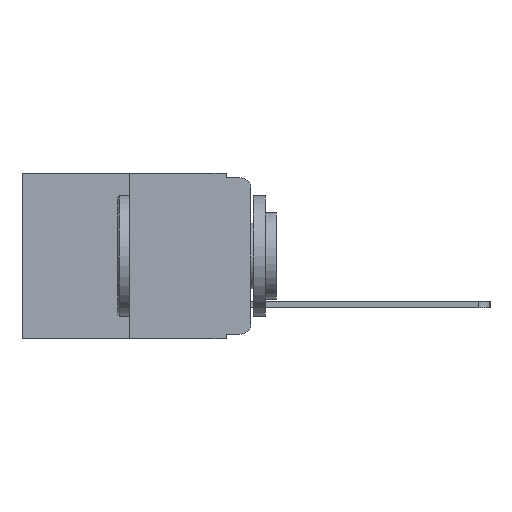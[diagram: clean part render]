
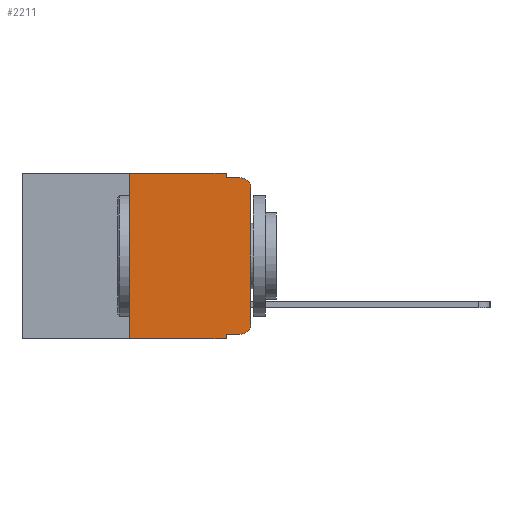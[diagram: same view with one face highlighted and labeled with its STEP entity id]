
A CAD part, left-side view. The second image highlights one B-rep face of the part: STEP entity #2211.
In plain terms, the highlighted planar face has unit normal (-1, 0, 0).
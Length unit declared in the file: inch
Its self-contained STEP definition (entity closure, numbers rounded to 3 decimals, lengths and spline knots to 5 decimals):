
#130 = CARTESIAN_POINT ( 'NONE',  ( 0., 0.473, 0. ) ) ;
#476 = DIRECTION ( 'NONE',  ( -1., 0., 0. ) ) ;
#540 = VECTOR ( 'NONE', #4897, 39.37008 ) ;
#891 = ORIENTED_EDGE ( 'NONE', *, *, #9728, .T. ) ;
#902 = LINE ( 'NONE', #9232, #6097 ) ;
#924 = VERTEX_POINT ( 'NONE', #2674 ) ;
#1056 = CIRCLE ( 'NONE', #1705, 0.02 ) ;
#1134 = VERTEX_POINT ( 'NONE', #9657 ) ;
#1220 = LINE ( 'NONE', #130, #8833 ) ;
#1580 = VECTOR ( 'NONE', #7499, 39.37008 ) ;
#1705 = AXIS2_PLACEMENT_3D ( 'NONE', #10366, #5227, #11197 ) ;
#1789 = DIRECTION ( 'NONE',  ( 0., 0., -1. ) ) ;
#2211 = ADVANCED_FACE ( 'NONE', ( #8863 ), #8914, .F. ) ;
#2260 = VECTOR ( 'NONE', #2673, 39.37008 ) ;
#2673 = DIRECTION ( 'NONE',  ( 0., 0., 1. ) ) ;
#2674 = CARTESIAN_POINT ( 'NONE',  ( 0., 0.051, -0.01 ) ) ;
#2981 = ORIENTED_EDGE ( 'NONE', *, *, #9771, .F. ) ;
#3163 = VECTOR ( 'NONE', #7651, 39.37008 ) ;
#3220 = VERTEX_POINT ( 'NONE', #5065 ) ;
#3433 = CARTESIAN_POINT ( 'NONE',  ( 0., 0.25, -0.343 ) ) ;
#3993 = CARTESIAN_POINT ( 'NONE',  ( 0., 0.051, 0. ) ) ;
#4006 = EDGE_LOOP ( 'NONE', ( #891, #9384, #2981, #10443, #7419, #5955, #8093, #11116, #12118, #6270 ) ) ;
#4471 = VERTEX_POINT ( 'NONE', #10386 ) ;
#4511 = DIRECTION ( 'NONE',  ( 0., -1., 0. ) ) ;
#4897 = DIRECTION ( 'NONE',  ( 0., 0., 1. ) ) ;
#4905 = AXIS2_PLACEMENT_3D ( 'NONE', #5896, #8942, #1789 ) ;
#5065 = CARTESIAN_POINT ( 'NONE',  ( 0., 0., -0.03 ) ) ;
#5227 = DIRECTION ( 'NONE',  ( -1., 0., 0. ) ) ;
#5720 = CARTESIAN_POINT ( 'NONE',  ( 0., 0., -0.313 ) ) ;
#5896 = CARTESIAN_POINT ( 'NONE',  ( 0., 0.473, 0. ) ) ;
#5947 = CARTESIAN_POINT ( 'NONE',  ( 0., 0.473, -0.343 ) ) ;
#5955 = ORIENTED_EDGE ( 'NONE', *, *, #9822, .F. ) ;
#6097 = VECTOR ( 'NONE', #10084, 39.37008 ) ;
#6189 = VERTEX_POINT ( 'NONE', #9207 ) ;
#6250 = LINE ( 'NONE', #5947, #10202 ) ;
#6270 = ORIENTED_EDGE ( 'NONE', *, *, #10074, .T. ) ;
#6642 = CARTESIAN_POINT ( 'NONE',  ( 0., 0.02, -0.03 ) ) ;
#6830 = DIRECTION ( 'NONE',  ( 0., -1., 0. ) ) ;
#7419 = ORIENTED_EDGE ( 'NONE', *, *, #10217, .F. ) ;
#7467 = DIRECTION ( 'NONE',  ( 0., 0., -1. ) ) ;
#7499 = DIRECTION ( 'NONE',  ( 0., -1., 0. ) ) ;
#7651 = DIRECTION ( 'NONE',  ( 0., 0., -1. ) ) ;
#7803 = CARTESIAN_POINT ( 'NONE',  ( 0., 0.051, -0.333 ) ) ;
#8093 = ORIENTED_EDGE ( 'NONE', *, *, #9259, .T. ) ;
#8179 = CARTESIAN_POINT ( 'NONE',  ( 0., 0.25, 0. ) ) ;
#8280 = CARTESIAN_POINT ( 'NONE',  ( 0., 0., 0. ) ) ;
#8461 = VECTOR ( 'NONE', #10334, 39.37008 ) ;
#8833 = VECTOR ( 'NONE', #4511, 39.37008 ) ;
#8841 = LINE ( 'NONE', #10008, #1580 ) ;
#8863 = FACE_OUTER_BOUND ( 'NONE', #4006, .T. ) ;
#8914 = PLANE ( 'NONE',  #4905 ) ;
#8942 = DIRECTION ( 'NONE',  ( 1., 0., 0. ) ) ;
#8961 = LINE ( 'NONE', #7803, #8461 ) ;
#9112 = CIRCLE ( 'NONE', #11901, 0.02 ) ;
#9207 = CARTESIAN_POINT ( 'NONE',  ( 0., 0.02, -0.01 ) ) ;
#9231 = VERTEX_POINT ( 'NONE', #3993 ) ;
#9232 = CARTESIAN_POINT ( 'NONE',  ( 0., 0.051, 0. ) ) ;
#9259 = EDGE_CURVE ( 'NONE', #10180, #9506, #6250, .T. ) ;
#9384 = ORIENTED_EDGE ( 'NONE', *, *, #9740, .T. ) ;
#9506 = VERTEX_POINT ( 'NONE', #10412 ) ;
#9657 = CARTESIAN_POINT ( 'NONE',  ( 0., 0.02, -0.333 ) ) ;
#9728 = EDGE_CURVE ( 'NONE', #10998, #3220, #12096, .T. ) ;
#9740 = EDGE_CURVE ( 'NONE', #3220, #6189, #9112, .T. ) ;
#9771 = EDGE_CURVE ( 'NONE', #924, #6189, #8841, .T. ) ;
#9809 = EDGE_CURVE ( 'NONE', #9231, #924, #902, .T. ) ;
#9822 = EDGE_CURVE ( 'NONE', #10180, #11132, #10315, .T. ) ;
#9885 = EDGE_CURVE ( 'NONE', #4471, #9506, #11972, .T. ) ;
#10008 = CARTESIAN_POINT ( 'NONE',  ( 0., 0.051, -0.01 ) ) ;
#10042 = EDGE_CURVE ( 'NONE', #4471, #1134, #8961, .T. ) ;
#10074 = EDGE_CURVE ( 'NONE', #1134, #10998, #1056, .T. ) ;
#10084 = DIRECTION ( 'NONE',  ( 0., 0., -1. ) ) ;
#10180 = VERTEX_POINT ( 'NONE', #3433 ) ;
#10202 = VECTOR ( 'NONE', #6830, 39.37008 ) ;
#10217 = EDGE_CURVE ( 'NONE', #11132, #9231, #1220, .T. ) ;
#10315 = LINE ( 'NONE', #11727, #540 ) ;
#10334 = DIRECTION ( 'NONE',  ( 0., -1., 0. ) ) ;
#10366 = CARTESIAN_POINT ( 'NONE',  ( 0., 0.02, -0.313 ) ) ;
#10386 = CARTESIAN_POINT ( 'NONE',  ( 0., 0.051, -0.333 ) ) ;
#10412 = CARTESIAN_POINT ( 'NONE',  ( 0., 0.051, -0.343 ) ) ;
#10443 = ORIENTED_EDGE ( 'NONE', *, *, #9809, .F. ) ;
#10998 = VERTEX_POINT ( 'NONE', #5720 ) ;
#11116 = ORIENTED_EDGE ( 'NONE', *, *, #9885, .F. ) ;
#11132 = VERTEX_POINT ( 'NONE', #8179 ) ;
#11197 = DIRECTION ( 'NONE',  ( 0., 0., -1. ) ) ;
#11727 = CARTESIAN_POINT ( 'NONE',  ( 0., 0.25, 0. ) ) ;
#11788 = CARTESIAN_POINT ( 'NONE',  ( 0., 0.051, 0. ) ) ;
#11901 = AXIS2_PLACEMENT_3D ( 'NONE', #6642, #476, #7467 ) ;
#11972 = LINE ( 'NONE', #11788, #3163 ) ;
#12096 = LINE ( 'NONE', #8280, #2260 ) ;
#12118 = ORIENTED_EDGE ( 'NONE', *, *, #10042, .T. ) ;
